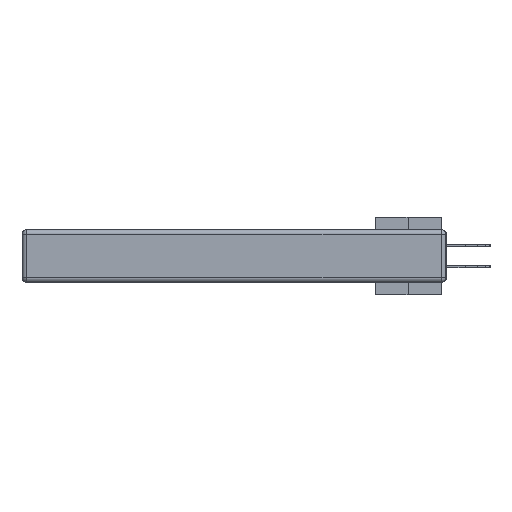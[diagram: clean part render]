
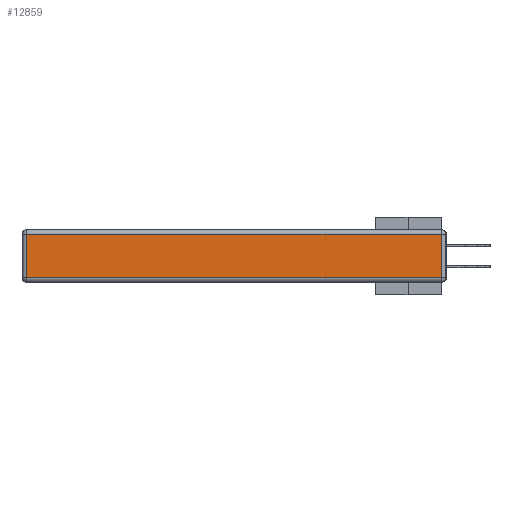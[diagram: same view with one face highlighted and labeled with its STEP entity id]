
A CAD part, left-side view. The second image highlights one B-rep face of the part: STEP entity #12859.
In plain terms, the highlighted planar face has unit normal (-1, 0, 0).
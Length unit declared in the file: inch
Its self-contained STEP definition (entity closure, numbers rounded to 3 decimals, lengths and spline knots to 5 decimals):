
#369 = FACE_OUTER_BOUND ( 'NONE', #23403, .T. ) ;
#2607 = CARTESIAN_POINT ( 'NONE',  ( 0., 0., -0.313 ) ) ;
#3153 = AXIS2_PLACEMENT_3D ( 'NONE', #14694, #4197, #21623 ) ;
#3810 = EDGE_CURVE ( 'NONE', #21415, #9872, #43946, .T. ) ;
#4197 = DIRECTION ( 'NONE',  ( -1., 0., 0. ) ) ;
#7658 = LINE ( 'NONE', #26346, #18940 ) ;
#9872 = VERTEX_POINT ( 'NONE', #25196 ) ;
#10667 = CARTESIAN_POINT ( 'NONE',  ( 0., 0.03, -0.313 ) ) ;
#12859 = ADVANCED_FACE ( 'NONE', ( #369 ), #14367, .T. ) ;
#14367 = PLANE ( 'NONE',  #3153 ) ;
#14694 = CARTESIAN_POINT ( 'NONE',  ( 0., 0., -0.343 ) ) ;
#15526 = DIRECTION ( 'NONE',  ( 0., 0., -1. ) ) ;
#18356 = EDGE_CURVE ( 'NONE', #9872, #40908, #7658, .T. ) ;
#18473 = EDGE_CURVE ( 'NONE', #40908, #18618, #37665, .T. ) ;
#18618 = VERTEX_POINT ( 'NONE', #10667 ) ;
#18940 = VECTOR ( 'NONE', #15526, 39.37008 ) ;
#19143 = ORIENTED_EDGE ( 'NONE', *, *, #23204, .T. ) ;
#21415 = VERTEX_POINT ( 'NONE', #26295 ) ;
#21623 = DIRECTION ( 'NONE',  ( 0., 0., 1. ) ) ;
#22131 = CARTESIAN_POINT ( 'NONE',  ( 0., 0.03, -0.343 ) ) ;
#23204 = EDGE_CURVE ( 'NONE', #18618, #21415, #32995, .T. ) ;
#23403 = EDGE_LOOP ( 'NONE', ( #41356, #19143, #43560, #39917 ) ) ;
#25196 = CARTESIAN_POINT ( 'NONE',  ( 0., 2.72, -0.03 ) ) ;
#25361 = VECTOR ( 'NONE', #27059, 39.37008 ) ;
#26295 = CARTESIAN_POINT ( 'NONE',  ( 0., 0.03, -0.03 ) ) ;
#26346 = CARTESIAN_POINT ( 'NONE',  ( 0., 2.72, -0.343 ) ) ;
#27059 = DIRECTION ( 'NONE',  ( 0., -1., 0. ) ) ;
#32031 = DIRECTION ( 'NONE',  ( 0., 1., 0. ) ) ;
#32995 = LINE ( 'NONE', #22131, #38871 ) ;
#34869 = VECTOR ( 'NONE', #32031, 39.37008 ) ;
#36217 = DIRECTION ( 'NONE',  ( 0., 0., 1. ) ) ;
#37665 = LINE ( 'NONE', #2607, #25361 ) ;
#38871 = VECTOR ( 'NONE', #36217, 39.37008 ) ;
#39917 = ORIENTED_EDGE ( 'NONE', *, *, #18356, .T. ) ;
#40536 = CARTESIAN_POINT ( 'NONE',  ( 0., 2.72, -0.313 ) ) ;
#40908 = VERTEX_POINT ( 'NONE', #40536 ) ;
#41356 = ORIENTED_EDGE ( 'NONE', *, *, #18473, .T. ) ;
#42194 = CARTESIAN_POINT ( 'NONE',  ( 0., 2.75, -0.03 ) ) ;
#43560 = ORIENTED_EDGE ( 'NONE', *, *, #3810, .T. ) ;
#43946 = LINE ( 'NONE', #42194, #34869 ) ;
